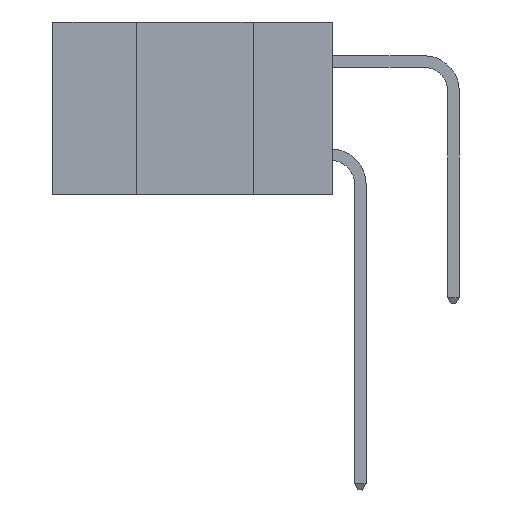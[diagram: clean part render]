
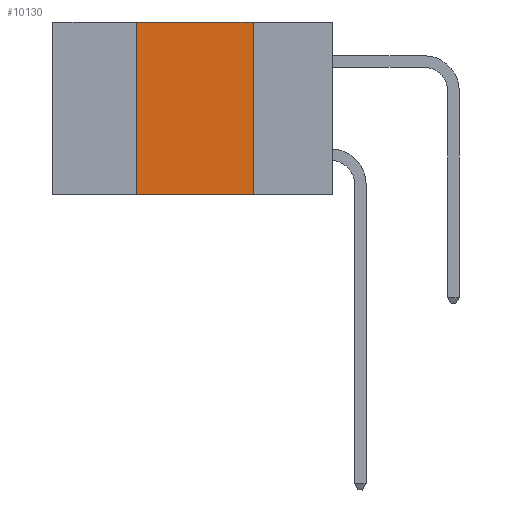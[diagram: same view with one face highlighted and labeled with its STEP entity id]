
A CAD part, left-side view. The second image highlights one B-rep face of the part: STEP entity #10130.
In plain terms, the highlighted planar face has unit normal (-1, 0, 0).
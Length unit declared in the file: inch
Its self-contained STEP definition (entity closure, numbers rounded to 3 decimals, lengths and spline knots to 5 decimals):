
#50 = PLANE ( 'NONE',  #4383 ) ;
#275 = EDGE_CURVE ( 'NONE', #12918, #12493, #10390, .T. ) ;
#639 = EDGE_CURVE ( 'NONE', #4658, #12493, #4270, .T. ) ;
#800 = DIRECTION ( 'NONE',  ( 0., -1., 0. ) ) ;
#1143 = VECTOR ( 'NONE', #1243, 39.37008 ) ;
#1153 = ORIENTED_EDGE ( 'NONE', *, *, #639, .F. ) ;
#1243 = DIRECTION ( 'NONE',  ( 0., -1., 0. ) ) ;
#1667 = CARTESIAN_POINT ( 'NONE',  ( 0., 0.17, 0. ) ) ;
#1878 = ORIENTED_EDGE ( 'NONE', *, *, #275, .T. ) ;
#2159 = VECTOR ( 'NONE', #800, 39.37008 ) ;
#2213 = DIRECTION ( 'NONE',  ( 0., 0., -1. ) ) ;
#2523 = LINE ( 'NONE', #11811, #6924 ) ;
#2711 = ORIENTED_EDGE ( 'NONE', *, *, #9548, .F. ) ;
#2791 = EDGE_CURVE ( 'NONE', #9646, #4658, #5861, .T. ) ;
#3021 = ORIENTED_EDGE ( 'NONE', *, *, #2791, .F. ) ;
#3150 = CARTESIAN_POINT ( 'NONE',  ( 0., 0.17, -0.37 ) ) ;
#3571 = VECTOR ( 'NONE', #2213, 39.37008 ) ;
#3913 = DIRECTION ( 'NONE',  ( 0., 0., -1. ) ) ;
#4039 = FACE_OUTER_BOUND ( 'NONE', #7975, .T. ) ;
#4105 = CARTESIAN_POINT ( 'NONE',  ( 0., 0.6, 0. ) ) ;
#4270 = LINE ( 'NONE', #3150, #3571 ) ;
#4383 = AXIS2_PLACEMENT_3D ( 'NONE', #4105, #11930, #3913 ) ;
#4658 = VERTEX_POINT ( 'NONE', #1667 ) ;
#5861 = LINE ( 'NONE', #9952, #2159 ) ;
#6097 = CARTESIAN_POINT ( 'NONE',  ( 0., 0.6, -0.37 ) ) ;
#6924 = VECTOR ( 'NONE', #12880, 39.37008 ) ;
#7975 = EDGE_LOOP ( 'NONE', ( #1153, #3021, #2711, #1878 ) ) ;
#9548 = EDGE_CURVE ( 'NONE', #12918, #9646, #2523, .T. ) ;
#9646 = VERTEX_POINT ( 'NONE', #12078 ) ;
#9952 = CARTESIAN_POINT ( 'NONE',  ( 0., 0.6, 0. ) ) ;
#10130 = ADVANCED_FACE ( 'NONE', ( #4039 ), #50, .F. ) ;
#10390 = LINE ( 'NONE', #6097, #1143 ) ;
#11811 = CARTESIAN_POINT ( 'NONE',  ( 0., 0.42, -0.37 ) ) ;
#11930 = DIRECTION ( 'NONE',  ( 1., 0., 0. ) ) ;
#11960 = CARTESIAN_POINT ( 'NONE',  ( 0., 0.17, -0.37 ) ) ;
#11995 = CARTESIAN_POINT ( 'NONE',  ( 0., 0.42, -0.37 ) ) ;
#12078 = CARTESIAN_POINT ( 'NONE',  ( 0., 0.42, 0. ) ) ;
#12493 = VERTEX_POINT ( 'NONE', #11960 ) ;
#12880 = DIRECTION ( 'NONE',  ( 0., 0., 1. ) ) ;
#12918 = VERTEX_POINT ( 'NONE', #11995 ) ;
